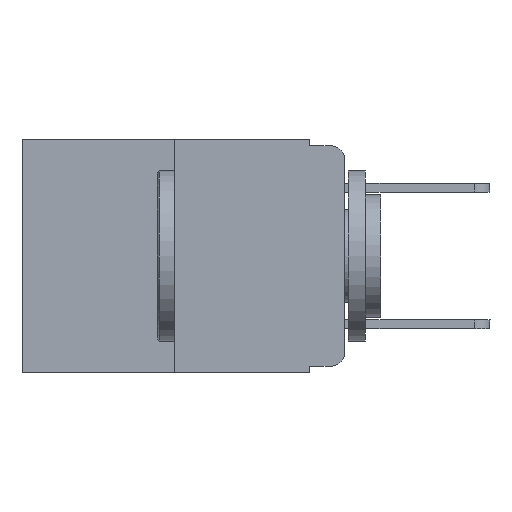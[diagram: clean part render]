
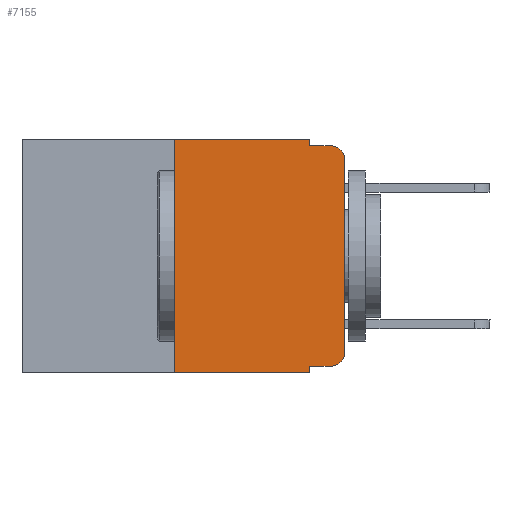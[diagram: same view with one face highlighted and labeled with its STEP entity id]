
A CAD part, left-side view. The second image highlights one B-rep face of the part: STEP entity #7155.
In plain terms, the highlighted planar face has unit normal (-1, 0, 0).
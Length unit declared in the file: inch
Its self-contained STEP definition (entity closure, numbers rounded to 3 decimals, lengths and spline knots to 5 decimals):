
#147 = DIRECTION ( 'NONE',  ( 1., 0., 0. ) ) ;
#310 = EDGE_CURVE ( 'NONE', #12769, #3648, #2701, .T. ) ;
#1685 = CARTESIAN_POINT ( 'NONE',  ( 0., 0.051, -0.343 ) ) ;
#1720 = ORIENTED_EDGE ( 'NONE', *, *, #15222, .T. ) ;
#1740 = VERTEX_POINT ( 'NONE', #21763 ) ;
#1804 = EDGE_CURVE ( 'NONE', #23359, #23462, #23581, .T. ) ;
#1943 = PLANE ( 'NONE',  #19860 ) ;
#2044 = CARTESIAN_POINT ( 'NONE',  ( 0., 0., -0.313 ) ) ;
#2270 = ORIENTED_EDGE ( 'NONE', *, *, #10244, .F. ) ;
#2409 = CARTESIAN_POINT ( 'NONE',  ( 0., 0.051, -0.333 ) ) ;
#2701 = LINE ( 'NONE', #9707, #20730 ) ;
#2922 = CARTESIAN_POINT ( 'NONE',  ( 0., 0.02, -0.333 ) ) ;
#3196 = VECTOR ( 'NONE', #10887, 39.37008 ) ;
#3648 = VERTEX_POINT ( 'NONE', #2922 ) ;
#4152 = DIRECTION ( 'NONE',  ( -1., 0., 0. ) ) ;
#4208 = DIRECTION ( 'NONE',  ( 0., 0., -1. ) ) ;
#4686 = DIRECTION ( 'NONE',  ( 0., 0., 1. ) ) ;
#5157 = CARTESIAN_POINT ( 'NONE',  ( 0., 0.051, 0. ) ) ;
#5303 = LINE ( 'NONE', #18194, #21900 ) ;
#5607 = VERTEX_POINT ( 'NONE', #2044 ) ;
#5746 = CARTESIAN_POINT ( 'NONE',  ( 0., 0., -0.03 ) ) ;
#6448 = DIRECTION ( 'NONE',  ( 0., -1., 0. ) ) ;
#6629 = VERTEX_POINT ( 'NONE', #5157 ) ;
#7070 = CARTESIAN_POINT ( 'NONE',  ( 0., 0., 0. ) ) ;
#7147 = LINE ( 'NONE', #16390, #12470 ) ;
#7155 = ADVANCED_FACE ( 'NONE', ( #23801 ), #1943, .F. ) ;
#7265 = DIRECTION ( 'NONE',  ( 0., 0., -1. ) ) ;
#7266 = EDGE_CURVE ( 'NONE', #3648, #5607, #18687, .T. ) ;
#7591 = EDGE_LOOP ( 'NONE', ( #1720, #14452, #2270, #18264, #15639, #17774, #17723, #16384, #11874, #19931 ) ) ;
#8336 = CARTESIAN_POINT ( 'NONE',  ( 0., 0.25, 0. ) ) ;
#8567 = VERTEX_POINT ( 'NONE', #12828 ) ;
#8879 = CARTESIAN_POINT ( 'NONE',  ( 0., 0.051, 0. ) ) ;
#9192 = AXIS2_PLACEMENT_3D ( 'NONE', #16701, #4152, #20443 ) ;
#9309 = CARTESIAN_POINT ( 'NONE',  ( 0., 0.473, 0. ) ) ;
#9395 = VERTEX_POINT ( 'NONE', #5746 ) ;
#9707 = CARTESIAN_POINT ( 'NONE',  ( 0., 0.051, -0.333 ) ) ;
#9803 = VERTEX_POINT ( 'NONE', #19715 ) ;
#10244 = EDGE_CURVE ( 'NONE', #9803, #8567, #17879, .T. ) ;
#10600 = LINE ( 'NONE', #8336, #10993 ) ;
#10773 = CARTESIAN_POINT ( 'NONE',  ( 0., 0.473, -0.343 ) ) ;
#10863 = VECTOR ( 'NONE', #16315, 39.37008 ) ;
#10887 = DIRECTION ( 'NONE',  ( 0., -1., 0. ) ) ;
#10993 = VECTOR ( 'NONE', #4686, 39.37008 ) ;
#11223 = CARTESIAN_POINT ( 'NONE',  ( 0., 0.02, -0.313 ) ) ;
#11368 = EDGE_CURVE ( 'NONE', #12769, #23462, #7147, .T. ) ;
#11874 = ORIENTED_EDGE ( 'NONE', *, *, #310, .T. ) ;
#12120 = LINE ( 'NONE', #7070, #20347 ) ;
#12470 = VECTOR ( 'NONE', #20146, 39.37008 ) ;
#12643 = DIRECTION ( 'NONE',  ( 0., -1., 0. ) ) ;
#12726 = VECTOR ( 'NONE', #17651, 39.37008 ) ;
#12769 = VERTEX_POINT ( 'NONE', #2409 ) ;
#12828 = CARTESIAN_POINT ( 'NONE',  ( 0., 0.02, -0.01 ) ) ;
#12901 = EDGE_CURVE ( 'NONE', #23359, #1740, #10600, .T. ) ;
#14452 = ORIENTED_EDGE ( 'NONE', *, *, #20984, .T. ) ;
#15222 = EDGE_CURVE ( 'NONE', #5607, #9395, #12120, .T. ) ;
#15639 = ORIENTED_EDGE ( 'NONE', *, *, #15668, .F. ) ;
#15668 = EDGE_CURVE ( 'NONE', #1740, #6629, #5303, .T. ) ;
#16315 = DIRECTION ( 'NONE',  ( 0., -1., 0. ) ) ;
#16384 = ORIENTED_EDGE ( 'NONE', *, *, #11368, .F. ) ;
#16390 = CARTESIAN_POINT ( 'NONE',  ( 0., 0.051, 0. ) ) ;
#16701 = CARTESIAN_POINT ( 'NONE',  ( 0., 0.02, -0.03 ) ) ;
#17651 = DIRECTION ( 'NONE',  ( 0., 0., -1. ) ) ;
#17723 = ORIENTED_EDGE ( 'NONE', *, *, #1804, .T. ) ;
#17774 = ORIENTED_EDGE ( 'NONE', *, *, #12901, .F. ) ;
#17779 = LINE ( 'NONE', #8879, #12726 ) ;
#17876 = EDGE_CURVE ( 'NONE', #6629, #9803, #17779, .T. ) ;
#17879 = LINE ( 'NONE', #19821, #3196 ) ;
#18194 = CARTESIAN_POINT ( 'NONE',  ( 0., 0.473, 0. ) ) ;
#18264 = ORIENTED_EDGE ( 'NONE', *, *, #17876, .F. ) ;
#18687 = CIRCLE ( 'NONE', #20238, 0.02 ) ;
#19471 = DIRECTION ( 'NONE',  ( 0., 0., 1. ) ) ;
#19715 = CARTESIAN_POINT ( 'NONE',  ( 0., 0.051, -0.01 ) ) ;
#19821 = CARTESIAN_POINT ( 'NONE',  ( 0., 0.051, -0.01 ) ) ;
#19860 = AXIS2_PLACEMENT_3D ( 'NONE', #9309, #147, #7265 ) ;
#19931 = ORIENTED_EDGE ( 'NONE', *, *, #7266, .T. ) ;
#20146 = DIRECTION ( 'NONE',  ( 0., 0., -1. ) ) ;
#20238 = AXIS2_PLACEMENT_3D ( 'NONE', #11223, #22565, #4208 ) ;
#20347 = VECTOR ( 'NONE', #19471, 39.37008 ) ;
#20443 = DIRECTION ( 'NONE',  ( 0., 0., -1. ) ) ;
#20728 = CIRCLE ( 'NONE', #9192, 0.02 ) ;
#20730 = VECTOR ( 'NONE', #6448, 39.37008 ) ;
#20984 = EDGE_CURVE ( 'NONE', #9395, #8567, #20728, .T. ) ;
#21688 = CARTESIAN_POINT ( 'NONE',  ( 0., 0.25, -0.343 ) ) ;
#21763 = CARTESIAN_POINT ( 'NONE',  ( 0., 0.25, 0. ) ) ;
#21900 = VECTOR ( 'NONE', #12643, 39.37008 ) ;
#22565 = DIRECTION ( 'NONE',  ( -1., 0., 0. ) ) ;
#23359 = VERTEX_POINT ( 'NONE', #21688 ) ;
#23462 = VERTEX_POINT ( 'NONE', #1685 ) ;
#23581 = LINE ( 'NONE', #10773, #10863 ) ;
#23801 = FACE_OUTER_BOUND ( 'NONE', #7591, .T. ) ;
